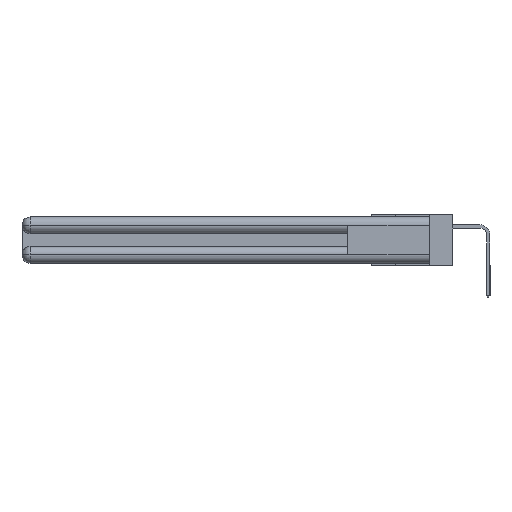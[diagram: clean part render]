
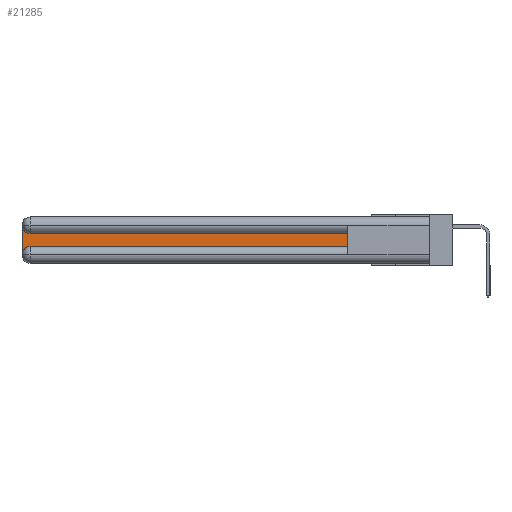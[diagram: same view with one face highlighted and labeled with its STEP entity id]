
A CAD part, left-side view. The second image highlights one B-rep face of the part: STEP entity #21285.
In plain terms, the highlighted planar face has unit normal (-1, 0, 0).
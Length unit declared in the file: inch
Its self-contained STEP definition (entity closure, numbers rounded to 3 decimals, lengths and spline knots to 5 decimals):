
#294 = VERTEX_POINT ( 'NONE', #26216 ) ;
#361 = DIRECTION ( 'NONE',  ( 0., 0., -1. ) ) ;
#1676 = LINE ( 'NONE', #15656, #24834 ) ;
#1921 = DIRECTION ( 'NONE',  ( 0., 0., 1. ) ) ;
#2298 = CARTESIAN_POINT ( 'NONE',  ( 0.075, 0.6, -0.1225 ) ) ;
#2963 = VERTEX_POINT ( 'NONE', #18601 ) ;
#3661 = CARTESIAN_POINT ( 'NONE',  ( 0.075, 3., -0.2175 ) ) ;
#4483 = EDGE_CURVE ( 'NONE', #7714, #19706, #11640, .T. ) ;
#5025 = AXIS2_PLACEMENT_3D ( 'NONE', #5061, #13253, #23285 ) ;
#5061 = CARTESIAN_POINT ( 'NONE',  ( 0.075, 2.94, -0.0625 ) ) ;
#6260 = ORIENTED_EDGE ( 'NONE', *, *, #10228, .T. ) ;
#6766 = CARTESIAN_POINT ( 'NONE',  ( 0.075, 0.6, -0.2175 ) ) ;
#7043 = LINE ( 'NONE', #3661, #20517 ) ;
#7186 = EDGE_CURVE ( 'NONE', #19706, #2963, #7043, .T. ) ;
#7714 = VERTEX_POINT ( 'NONE', #21105 ) ;
#8305 = CARTESIAN_POINT ( 'NONE',  ( 0.075, 0.6, -0.2175 ) ) ;
#8489 = EDGE_LOOP ( 'NONE', ( #6260, #18146, #21138, #17506, #14854, #15637 ) ) ;
#9804 = LINE ( 'NONE', #2298, #20705 ) ;
#10228 = EDGE_CURVE ( 'NONE', #294, #7714, #9804, .T. ) ;
#10347 = CARTESIAN_POINT ( 'NONE',  ( 0.075, 3., -0.0625 ) ) ;
#10677 = DIRECTION ( 'NONE',  ( 0., 1., 0. ) ) ;
#11133 = PLANE ( 'NONE',  #11326 ) ;
#11326 = AXIS2_PLACEMENT_3D ( 'NONE', #15276, #21698, #13114 ) ;
#11640 = CIRCLE ( 'NONE', #5025, 0.06 ) ;
#11859 = VECTOR ( 'NONE', #1921, 39.37008 ) ;
#12141 = LINE ( 'NONE', #8305, #11859 ) ;
#12952 = FACE_OUTER_BOUND ( 'NONE', #8489, .T. ) ;
#13114 = DIRECTION ( 'NONE',  ( 0., 0., -1. ) ) ;
#13253 = DIRECTION ( 'NONE',  ( 1., 0., 0. ) ) ;
#13760 = DIRECTION ( 'NONE',  ( 0., -1., 0. ) ) ;
#13776 = AXIS2_PLACEMENT_3D ( 'NONE', #23057, #16977, #361 ) ;
#14117 = VERTEX_POINT ( 'NONE', #24873 ) ;
#14854 = ORIENTED_EDGE ( 'NONE', *, *, #18791, .T. ) ;
#15162 = CIRCLE ( 'NONE', #13776, 0.06 ) ;
#15276 = CARTESIAN_POINT ( 'NONE',  ( 0.075, 3., -0.1225 ) ) ;
#15600 = VERTEX_POINT ( 'NONE', #6766 ) ;
#15637 = ORIENTED_EDGE ( 'NONE', *, *, #16083, .T. ) ;
#15656 = CARTESIAN_POINT ( 'NONE',  ( 0.075, 0.6, -0.2175 ) ) ;
#16083 = EDGE_CURVE ( 'NONE', #15600, #294, #12141, .T. ) ;
#16977 = DIRECTION ( 'NONE',  ( 1., 0., 0. ) ) ;
#17506 = ORIENTED_EDGE ( 'NONE', *, *, #22321, .T. ) ;
#18146 = ORIENTED_EDGE ( 'NONE', *, *, #4483, .T. ) ;
#18601 = CARTESIAN_POINT ( 'NONE',  ( 0.075, 3., -0.2775 ) ) ;
#18791 = EDGE_CURVE ( 'NONE', #14117, #15600, #1676, .T. ) ;
#19706 = VERTEX_POINT ( 'NONE', #10347 ) ;
#20517 = VECTOR ( 'NONE', #21777, 39.37008 ) ;
#20705 = VECTOR ( 'NONE', #10677, 39.37008 ) ;
#21105 = CARTESIAN_POINT ( 'NONE',  ( 0.075, 2.94, -0.1225 ) ) ;
#21138 = ORIENTED_EDGE ( 'NONE', *, *, #7186, .T. ) ;
#21285 = ADVANCED_FACE ( 'NONE', ( #12952 ), #11133, .F. ) ;
#21698 = DIRECTION ( 'NONE',  ( 1., 0., 0. ) ) ;
#21777 = DIRECTION ( 'NONE',  ( 0., 0., -1. ) ) ;
#22321 = EDGE_CURVE ( 'NONE', #2963, #14117, #15162, .T. ) ;
#23057 = CARTESIAN_POINT ( 'NONE',  ( 0.075, 2.94, -0.2775 ) ) ;
#23285 = DIRECTION ( 'NONE',  ( 0., 0., -1. ) ) ;
#24834 = VECTOR ( 'NONE', #13760, 39.37008 ) ;
#24873 = CARTESIAN_POINT ( 'NONE',  ( 0.075, 2.94, -0.2175 ) ) ;
#26216 = CARTESIAN_POINT ( 'NONE',  ( 0.075, 0.6, -0.1225 ) ) ;
